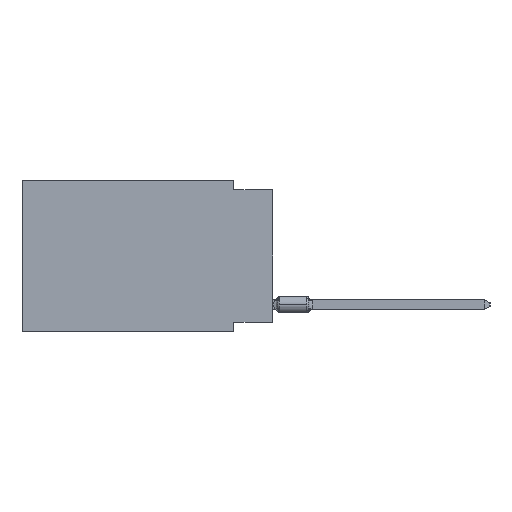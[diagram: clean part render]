
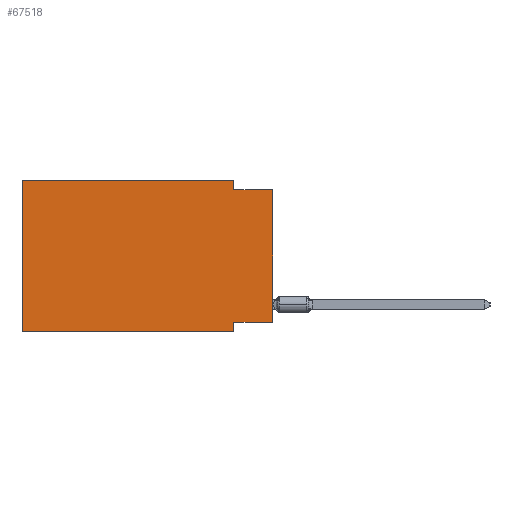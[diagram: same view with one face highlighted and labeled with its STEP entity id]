
A CAD part, left-side view. The second image highlights one B-rep face of the part: STEP entity #67518.
In plain terms, the highlighted planar face has unit normal (-1, 0, 0).
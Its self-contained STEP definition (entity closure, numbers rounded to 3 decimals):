
#1516 = DIRECTION ( 'NONE',  ( 1., 0., 0. ) ) ;
#3229 = DIRECTION ( 'NONE',  ( 0., 0., 1. ) ) ;
#3701 = EDGE_CURVE ( 'NONE', #28277, #8784, #20568, .T. ) ;
#4946 = VERTEX_POINT ( 'NONE', #10572 ) ;
#5889 = CARTESIAN_POINT ( 'NONE',  ( 0., 0., -0.635 ) ) ;
#8784 = VERTEX_POINT ( 'NONE', #29851 ) ;
#10572 = CARTESIAN_POINT ( 'NONE',  ( 0., 2.54, 0. ) ) ;
#11252 = VECTOR ( 'NONE', #3229, 1000. ) ;
#11641 = VECTOR ( 'NONE', #32364, 1000. ) ;
#12599 = DIRECTION ( 'NONE',  ( 0., 0., -1. ) ) ;
#12602 = LINE ( 'NONE', #24036, #52468 ) ;
#13590 = LINE ( 'NONE', #47565, #70472 ) ;
#13752 = EDGE_CURVE ( 'NONE', #16267, #53226, #12602, .T. ) ;
#16071 = LINE ( 'NONE', #31601, #36830 ) ;
#16267 = VERTEX_POINT ( 'NONE', #55290 ) ;
#17018 = ORIENTED_EDGE ( 'NONE', *, *, #42322, .T. ) ;
#17263 = CARTESIAN_POINT ( 'NONE',  ( 0., 2.54, -9.906 ) ) ;
#17810 = EDGE_CURVE ( 'NONE', #4946, #33747, #22997, .T. ) ;
#19249 = FACE_OUTER_BOUND ( 'NONE', #69210, .T. ) ;
#19482 = ORIENTED_EDGE ( 'NONE', *, *, #3701, .F. ) ;
#19845 = CARTESIAN_POINT ( 'NONE',  ( 0., 16.383, 0. ) ) ;
#20536 = CARTESIAN_POINT ( 'NONE',  ( 0., 2.54, -9.906 ) ) ;
#20568 = LINE ( 'NONE', #19845, #11252 ) ;
#20911 = DIRECTION ( 'NONE',  ( 0., 0., 1. ) ) ;
#22997 = LINE ( 'NONE', #62545, #11641 ) ;
#23872 = ORIENTED_EDGE ( 'NONE', *, *, #50919, .F. ) ;
#24036 = CARTESIAN_POINT ( 'NONE',  ( 0., 0., -9.271 ) ) ;
#25343 = ORIENTED_EDGE ( 'NONE', *, *, #17810, .F. ) ;
#26125 = VERTEX_POINT ( 'NONE', #20536 ) ;
#26784 = DIRECTION ( 'NONE',  ( 0., -1., 0. ) ) ;
#28277 = VERTEX_POINT ( 'NONE', #63192 ) ;
#28791 = ORIENTED_EDGE ( 'NONE', *, *, #34530, .F. ) ;
#29583 = DIRECTION ( 'NONE',  ( 0., 1., 0. ) ) ;
#29851 = CARTESIAN_POINT ( 'NONE',  ( 0., 16.383, 0. ) ) ;
#29954 = CARTESIAN_POINT ( 'NONE',  ( 0., 16.383, 0. ) ) ;
#31601 = CARTESIAN_POINT ( 'NONE',  ( 0., 0., -0.635 ) ) ;
#32220 = AXIS2_PLACEMENT_3D ( 'NONE', #29954, #1516, #12599 ) ;
#32364 = DIRECTION ( 'NONE',  ( 0., 0., -1. ) ) ;
#33245 = DIRECTION ( 'NONE',  ( 0., -1., 0. ) ) ;
#33509 = LINE ( 'NONE', #17263, #54231 ) ;
#33747 = VERTEX_POINT ( 'NONE', #38593 ) ;
#34241 = DIRECTION ( 'NONE',  ( 0., 0., -1. ) ) ;
#34530 = EDGE_CURVE ( 'NONE', #53226, #26125, #33509, .T. ) ;
#36830 = VECTOR ( 'NONE', #26784, 1000. ) ;
#38593 = CARTESIAN_POINT ( 'NONE',  ( 0., 2.54, -0.635 ) ) ;
#40239 = EDGE_CURVE ( 'NONE', #8784, #4946, #60999, .T. ) ;
#42322 = EDGE_CURVE ( 'NONE', #16267, #69356, #60808, .T. ) ;
#45490 = EDGE_CURVE ( 'NONE', #28277, #26125, #13590, .T. ) ;
#46983 = ORIENTED_EDGE ( 'NONE', *, *, #40239, .F. ) ;
#47565 = CARTESIAN_POINT ( 'NONE',  ( 0., 16.383, -9.906 ) ) ;
#47717 = VECTOR ( 'NONE', #20911, 1000. ) ;
#49170 = CARTESIAN_POINT ( 'NONE',  ( 0., 16.383, 0. ) ) ;
#50919 = EDGE_CURVE ( 'NONE', #33747, #69356, #16071, .T. ) ;
#52468 = VECTOR ( 'NONE', #29583, 1000. ) ;
#52734 = DIRECTION ( 'NONE',  ( 0., -1., 0. ) ) ;
#53226 = VERTEX_POINT ( 'NONE', #70433 ) ;
#54231 = VECTOR ( 'NONE', #34241, 1000. ) ;
#54940 = ORIENTED_EDGE ( 'NONE', *, *, #13752, .F. ) ;
#55290 = CARTESIAN_POINT ( 'NONE',  ( 0., 0., -9.271 ) ) ;
#58606 = ORIENTED_EDGE ( 'NONE', *, *, #45490, .T. ) ;
#59390 = VECTOR ( 'NONE', #33245, 1000. ) ;
#60808 = LINE ( 'NONE', #72264, #47717 ) ;
#60999 = LINE ( 'NONE', #49170, #59390 ) ;
#62545 = CARTESIAN_POINT ( 'NONE',  ( 0., 2.54, 0. ) ) ;
#63192 = CARTESIAN_POINT ( 'NONE',  ( 0., 16.383, -9.906 ) ) ;
#67518 = ADVANCED_FACE ( 'NONE', ( #19249 ), #68765, .F. ) ;
#68765 = PLANE ( 'NONE',  #32220 ) ;
#69210 = EDGE_LOOP ( 'NONE', ( #17018, #23872, #25343, #46983, #19482, #58606, #28791, #54940 ) ) ;
#69356 = VERTEX_POINT ( 'NONE', #5889 ) ;
#70433 = CARTESIAN_POINT ( 'NONE',  ( 0., 2.54, -9.271 ) ) ;
#70472 = VECTOR ( 'NONE', #52734, 1000. ) ;
#72264 = CARTESIAN_POINT ( 'NONE',  ( 0., 0., 0. ) ) ;
